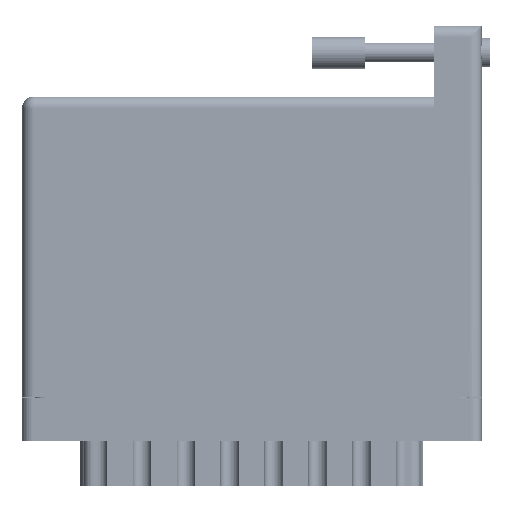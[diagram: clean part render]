
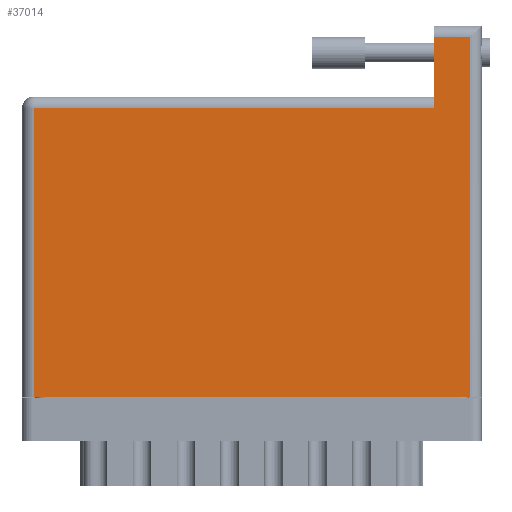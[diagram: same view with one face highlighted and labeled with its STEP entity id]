
A CAD part, front view. The second image highlights one B-rep face of the part: STEP entity #37014.
In plain terms, the highlighted face is planar.
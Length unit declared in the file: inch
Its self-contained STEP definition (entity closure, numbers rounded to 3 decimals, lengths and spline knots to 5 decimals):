
#188 = LINE ( 'NONE', #10377, #40647 ) ;
#698 = DIRECTION ( 'NONE',  ( -1., 0., 0. ) ) ;
#3850 = EDGE_CURVE ( 'NONE', #64252, #64348, #188, .T. ) ;
#7678 = DIRECTION ( 'NONE',  ( -1., 0., 0. ) ) ;
#7919 = CARTESIAN_POINT ( 'NONE',  ( 0., 1.775, 0. ) ) ;
#10377 = CARTESIAN_POINT ( 'NONE',  ( 0., 1.705, 0. ) ) ;
#10704 = ORIENTED_EDGE ( 'NONE', *, *, #46849, .T. ) ;
#10852 = EDGE_CURVE ( 'NONE', #59719, #35207, #15823, .T. ) ;
#12337 = CARTESIAN_POINT ( 'NONE',  ( 0.07, 1.705, 0. ) ) ;
#12697 = AXIS2_PLACEMENT_3D ( 'NONE', #7919, #69504, #7678 ) ;
#13057 = CARTESIAN_POINT ( 'NONE',  ( 2.438, 2.125, 0. ) ) ;
#15823 = LINE ( 'NONE', #34122, #18434 ) ;
#16230 = CARTESIAN_POINT ( 'NONE',  ( 2.438, 2.195, 0. ) ) ;
#18434 = VECTOR ( 'NONE', #698, 39.37008 ) ;
#19682 = VECTOR ( 'NONE', #37177, 39.37008 ) ;
#20487 = DIRECTION ( 'NONE',  ( -1., 0., 0. ) ) ;
#22978 = VERTEX_POINT ( 'NONE', #64514 ) ;
#23132 = VECTOR ( 'NONE', #43914, 39.37008 ) ;
#26382 = ORIENTED_EDGE ( 'NONE', *, *, #10852, .T. ) ;
#28847 = ORIENTED_EDGE ( 'NONE', *, *, #60258, .T. ) ;
#30772 = PLANE ( 'NONE',  #12697 ) ;
#33195 = DIRECTION ( 'NONE',  ( 0., -1., 0. ) ) ;
#33518 = CARTESIAN_POINT ( 'NONE',  ( 2.648, 2.125, 0. ) ) ;
#34122 = CARTESIAN_POINT ( 'NONE',  ( 0., 2.125, 0. ) ) ;
#34987 = VECTOR ( 'NONE', #44622, 39.37008 ) ;
#35207 = VERTEX_POINT ( 'NONE', #13057 ) ;
#37014 = ADVANCED_FACE ( 'NONE', ( #55788 ), #30772, .F. ) ;
#37177 = DIRECTION ( 'NONE',  ( 0., -1., 0. ) ) ;
#37193 = LINE ( 'NONE', #38065, #23132 ) ;
#38065 = CARTESIAN_POINT ( 'NONE',  ( 2.648, 2.195, 0. ) ) ;
#40647 = VECTOR ( 'NONE', #20487, 39.37008 ) ;
#42073 = CARTESIAN_POINT ( 'NONE',  ( 0.07, 0., 0. ) ) ;
#43914 = DIRECTION ( 'NONE',  ( 0., 1., 0. ) ) ;
#44622 = DIRECTION ( 'NONE',  ( 1., 0., 0. ) ) ;
#46849 = EDGE_CURVE ( 'NONE', #70067, #22978, #49861, .T. ) ;
#47385 = ORIENTED_EDGE ( 'NONE', *, *, #3850, .T. ) ;
#49861 = LINE ( 'NONE', #71130, #34987 ) ;
#49921 = LINE ( 'NONE', #16230, #60478 ) ;
#55788 = FACE_OUTER_BOUND ( 'NONE', #63063, .T. ) ;
#56235 = CARTESIAN_POINT ( 'NONE',  ( 2.438, 1.705, 0. ) ) ;
#57466 = EDGE_CURVE ( 'NONE', #64348, #70067, #67955, .T. ) ;
#59719 = VERTEX_POINT ( 'NONE', #33518 ) ;
#59881 = ORIENTED_EDGE ( 'NONE', *, *, #69266, .T. ) ;
#60258 = EDGE_CURVE ( 'NONE', #35207, #64252, #49921, .T. ) ;
#60478 = VECTOR ( 'NONE', #33195, 39.37008 ) ;
#63063 = EDGE_LOOP ( 'NONE', ( #47385, #70239, #10704, #59881, #26382, #28847 ) ) ;
#64252 = VERTEX_POINT ( 'NONE', #56235 ) ;
#64348 = VERTEX_POINT ( 'NONE', #12337 ) ;
#64514 = CARTESIAN_POINT ( 'NONE',  ( 2.648, 0., 0. ) ) ;
#67955 = LINE ( 'NONE', #42073, #19682 ) ;
#69266 = EDGE_CURVE ( 'NONE', #22978, #59719, #37193, .T. ) ;
#69504 = DIRECTION ( 'NONE',  ( 0., 0., -1. ) ) ;
#70067 = VERTEX_POINT ( 'NONE', #72736 ) ;
#70239 = ORIENTED_EDGE ( 'NONE', *, *, #57466, .T. ) ;
#71130 = CARTESIAN_POINT ( 'NONE',  ( 0., 0., 0. ) ) ;
#72736 = CARTESIAN_POINT ( 'NONE',  ( 0.07, 0., 0. ) ) ;
